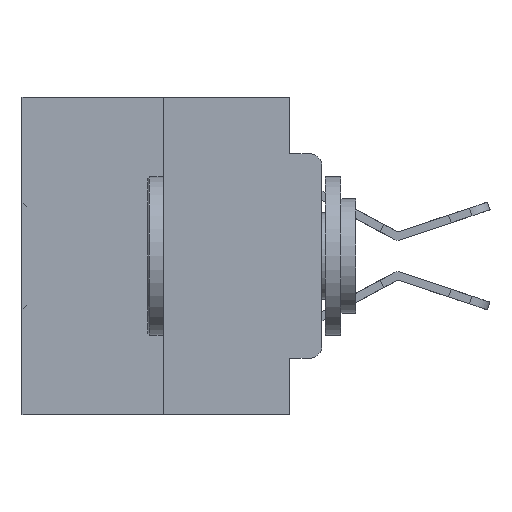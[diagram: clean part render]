
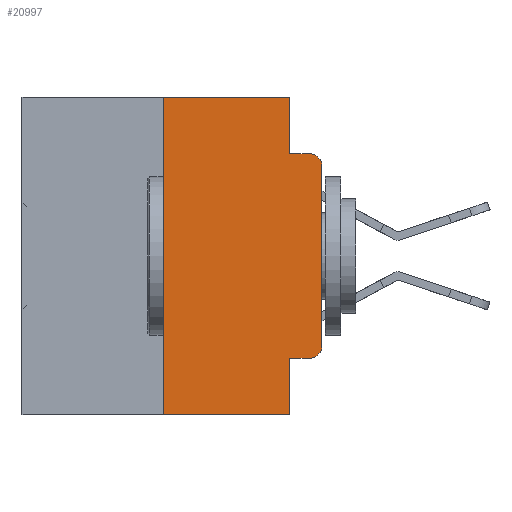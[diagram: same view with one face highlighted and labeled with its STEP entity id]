
A CAD part, left-side view. The second image highlights one B-rep face of the part: STEP entity #20997.
In plain terms, the highlighted planar face has unit normal (-1, 0, 0).
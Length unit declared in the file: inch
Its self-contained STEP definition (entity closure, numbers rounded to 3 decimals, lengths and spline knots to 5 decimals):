
#94 = CARTESIAN_POINT ( 'NONE',  ( 0., 0., 0. ) ) ;
#144 = DIRECTION ( 'NONE',  ( 0., 0., -1. ) ) ;
#272 = LINE ( 'NONE', #31959, #6735 ) ;
#882 = CARTESIAN_POINT ( 'NONE',  ( 0., 0.25, 0. ) ) ;
#2016 = EDGE_CURVE ( 'NONE', #26027, #3342, #32239, .T. ) ;
#2786 = DIRECTION ( 'NONE',  ( 0., 0., 1. ) ) ;
#3342 = VERTEX_POINT ( 'NONE', #18226 ) ;
#3775 = VECTOR ( 'NONE', #2786, 39.37008 ) ;
#3822 = LINE ( 'NONE', #16433, #26931 ) ;
#4256 = EDGE_CURVE ( 'NONE', #19213, #17603, #22203, .T. ) ;
#4412 = AXIS2_PLACEMENT_3D ( 'NONE', #7722, #26458, #10407 ) ;
#4657 = ORIENTED_EDGE ( 'NONE', *, *, #4256, .T. ) ;
#5075 = LINE ( 'NONE', #94, #11390 ) ;
#6068 = VERTEX_POINT ( 'NONE', #26136 ) ;
#6147 = CARTESIAN_POINT ( 'NONE',  ( 0., 0.473, 0. ) ) ;
#6331 = CIRCLE ( 'NONE', #20428, 0.02 ) ;
#6586 = DIRECTION ( 'NONE',  ( -1., 0., 0. ) ) ;
#6723 = LINE ( 'NONE', #17676, #33424 ) ;
#6735 = VECTOR ( 'NONE', #10622, 39.37008 ) ;
#7673 = LINE ( 'NONE', #28777, #21162 ) ;
#7722 = CARTESIAN_POINT ( 'NONE',  ( 0., 0.02, -0.3915 ) ) ;
#8748 = CARTESIAN_POINT ( 'NONE',  ( 0., 0.02, -0.4115 ) ) ;
#8971 = DIRECTION ( 'NONE',  ( 0., 0., -1. ) ) ;
#9602 = AXIS2_PLACEMENT_3D ( 'NONE', #6147, #25045, #8971 ) ;
#10192 = EDGE_CURVE ( 'NONE', #16016, #6068, #3822, .T. ) ;
#10407 = DIRECTION ( 'NONE',  ( 0., 0., -1. ) ) ;
#10622 = DIRECTION ( 'NONE',  ( 0., -1., 0. ) ) ;
#10864 = EDGE_CURVE ( 'NONE', #17603, #13643, #5075, .T. ) ;
#11069 = EDGE_CURVE ( 'NONE', #13643, #14095, #6331, .T. ) ;
#11390 = VECTOR ( 'NONE', #19126, 39.37008 ) ;
#11557 = PLANE ( 'NONE',  #9602 ) ;
#12220 = ORIENTED_EDGE ( 'NONE', *, *, #10192, .F. ) ;
#12810 = FACE_OUTER_BOUND ( 'NONE', #20144, .T. ) ;
#13484 = LINE ( 'NONE', #33649, #27715 ) ;
#13643 = VERTEX_POINT ( 'NONE', #32696 ) ;
#14095 = VERTEX_POINT ( 'NONE', #29361 ) ;
#14603 = CARTESIAN_POINT ( 'NONE',  ( 0., 0.051, -0.5 ) ) ;
#14646 = EDGE_CURVE ( 'NONE', #6068, #14095, #272, .T. ) ;
#15163 = VERTEX_POINT ( 'NONE', #23541 ) ;
#15184 = EDGE_CURVE ( 'NONE', #15163, #19213, #24757, .T. ) ;
#15272 = CARTESIAN_POINT ( 'NONE',  ( 0., 0.25, -0.5 ) ) ;
#15973 = VECTOR ( 'NONE', #28951, 39.37008 ) ;
#16016 = VERTEX_POINT ( 'NONE', #29197 ) ;
#16433 = CARTESIAN_POINT ( 'NONE',  ( 0., 0.051, 0. ) ) ;
#17603 = VERTEX_POINT ( 'NONE', #22639 ) ;
#17676 = CARTESIAN_POINT ( 'NONE',  ( 0., 0.473, 0. ) ) ;
#18223 = ORIENTED_EDGE ( 'NONE', *, *, #15184, .T. ) ;
#18226 = CARTESIAN_POINT ( 'NONE',  ( 0., 0.25, 0. ) ) ;
#18624 = ORIENTED_EDGE ( 'NONE', *, *, #22546, .T. ) ;
#18986 = ORIENTED_EDGE ( 'NONE', *, *, #10864, .T. ) ;
#19126 = DIRECTION ( 'NONE',  ( 0., 0., 1. ) ) ;
#19213 = VERTEX_POINT ( 'NONE', #8748 ) ;
#20144 = EDGE_LOOP ( 'NONE', ( #18986, #33029, #25667, #12220, #29373, #31023, #18624, #28981, #18223, #4657 ) ) ;
#20428 = AXIS2_PLACEMENT_3D ( 'NONE', #22717, #6586, #25388 ) ;
#20997 = ADVANCED_FACE ( 'NONE', ( #12810 ), #11557, .F. ) ;
#21162 = VECTOR ( 'NONE', #31409, 39.37008 ) ;
#22203 = CIRCLE ( 'NONE', #4412, 0.02 ) ;
#22546 = EDGE_CURVE ( 'NONE', #26027, #32210, #7673, .T. ) ;
#22639 = CARTESIAN_POINT ( 'NONE',  ( 0., 0., -0.3915 ) ) ;
#22717 = CARTESIAN_POINT ( 'NONE',  ( 0., 0.02, -0.1085 ) ) ;
#23541 = CARTESIAN_POINT ( 'NONE',  ( 0., 0.051, -0.4115 ) ) ;
#24757 = LINE ( 'NONE', #26291, #15973 ) ;
#25045 = DIRECTION ( 'NONE',  ( 1., 0., 0. ) ) ;
#25388 = DIRECTION ( 'NONE',  ( 0., 0., -1. ) ) ;
#25667 = ORIENTED_EDGE ( 'NONE', *, *, #14646, .F. ) ;
#25715 = DIRECTION ( 'NONE',  ( 0., -1., 0. ) ) ;
#26027 = VERTEX_POINT ( 'NONE', #15272 ) ;
#26136 = CARTESIAN_POINT ( 'NONE',  ( 0., 0.051, -0.0885 ) ) ;
#26291 = CARTESIAN_POINT ( 'NONE',  ( 0., 0.051, -0.4115 ) ) ;
#26458 = DIRECTION ( 'NONE',  ( -1., 0., 0. ) ) ;
#26931 = VECTOR ( 'NONE', #144, 39.37008 ) ;
#27715 = VECTOR ( 'NONE', #28383, 39.37008 ) ;
#28383 = DIRECTION ( 'NONE',  ( 0., 0., -1. ) ) ;
#28777 = CARTESIAN_POINT ( 'NONE',  ( 0., 0.473, -0.5 ) ) ;
#28951 = DIRECTION ( 'NONE',  ( 0., -1., 0. ) ) ;
#28981 = ORIENTED_EDGE ( 'NONE', *, *, #30348, .F. ) ;
#29197 = CARTESIAN_POINT ( 'NONE',  ( 0., 0.051, 0. ) ) ;
#29361 = CARTESIAN_POINT ( 'NONE',  ( 0., 0.02, -0.0885 ) ) ;
#29373 = ORIENTED_EDGE ( 'NONE', *, *, #30972, .F. ) ;
#30348 = EDGE_CURVE ( 'NONE', #15163, #32210, #13484, .T. ) ;
#30972 = EDGE_CURVE ( 'NONE', #3342, #16016, #6723, .T. ) ;
#31023 = ORIENTED_EDGE ( 'NONE', *, *, #2016, .F. ) ;
#31409 = DIRECTION ( 'NONE',  ( 0., -1., 0. ) ) ;
#31959 = CARTESIAN_POINT ( 'NONE',  ( 0., 0.051, -0.0885 ) ) ;
#32210 = VERTEX_POINT ( 'NONE', #14603 ) ;
#32239 = LINE ( 'NONE', #882, #3775 ) ;
#32696 = CARTESIAN_POINT ( 'NONE',  ( 0., 0., -0.1085 ) ) ;
#33029 = ORIENTED_EDGE ( 'NONE', *, *, #11069, .T. ) ;
#33424 = VECTOR ( 'NONE', #25715, 39.37008 ) ;
#33649 = CARTESIAN_POINT ( 'NONE',  ( 0., 0.051, 0. ) ) ;
